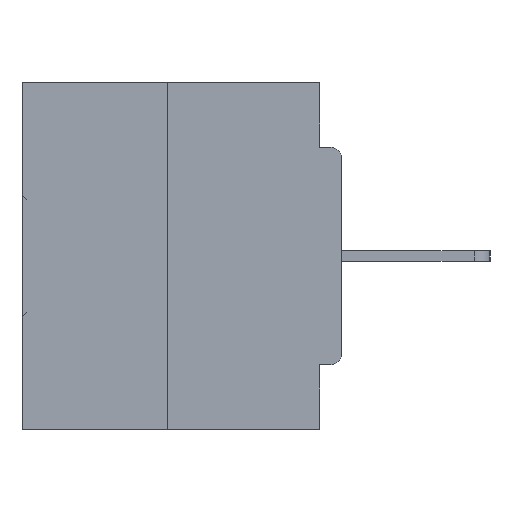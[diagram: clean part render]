
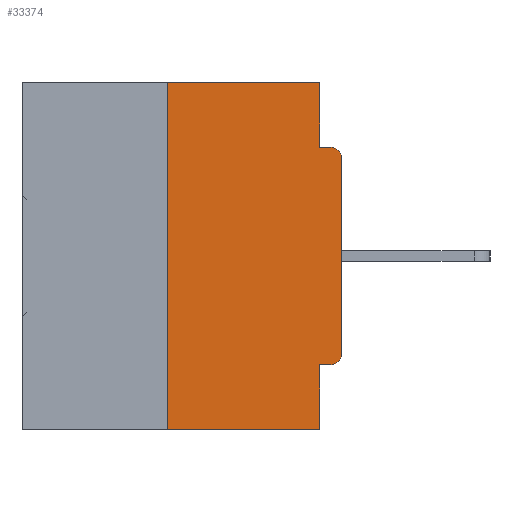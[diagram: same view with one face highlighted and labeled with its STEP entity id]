
A CAD part, left-side view. The second image highlights one B-rep face of the part: STEP entity #33374.
In plain terms, the highlighted planar face has unit normal (-1, 0, 0).
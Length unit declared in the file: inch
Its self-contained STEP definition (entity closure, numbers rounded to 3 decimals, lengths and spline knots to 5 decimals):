
#605 = LINE ( 'NONE', #21622, #7259 ) ;
#720 = EDGE_LOOP ( 'NONE', ( #32181, #9084, #12952, #34622, #1567, #32284, #33126, #6703, #37884, #9735 ) ) ;
#1174 = AXIS2_PLACEMENT_3D ( 'NONE', #32685, #8380, #14907 ) ;
#1273 = EDGE_CURVE ( 'NONE', #7712, #2412, #1544, .T. ) ;
#1544 = LINE ( 'NONE', #19913, #4070 ) ;
#1567 = ORIENTED_EDGE ( 'NONE', *, *, #1273, .F. ) ;
#2412 = VERTEX_POINT ( 'NONE', #40136 ) ;
#3053 = DIRECTION ( 'NONE',  ( 0., 0., -1. ) ) ;
#3484 = VERTEX_POINT ( 'NONE', #8749 ) ;
#3762 = CARTESIAN_POINT ( 'NONE',  ( 0., 0., 0. ) ) ;
#4070 = VECTOR ( 'NONE', #16831, 39.37008 ) ;
#6509 = CARTESIAN_POINT ( 'NONE',  ( 0., 0.031, 0. ) ) ;
#6703 = ORIENTED_EDGE ( 'NONE', *, *, #16996, .T. ) ;
#6751 = VERTEX_POINT ( 'NONE', #17397 ) ;
#7259 = VECTOR ( 'NONE', #18579, 39.37008 ) ;
#7712 = VERTEX_POINT ( 'NONE', #39703 ) ;
#8380 = DIRECTION ( 'NONE',  ( -1., 0., 0. ) ) ;
#8749 = CARTESIAN_POINT ( 'NONE',  ( 0., 0., -0.3915 ) ) ;
#9084 = ORIENTED_EDGE ( 'NONE', *, *, #36706, .F. ) ;
#9555 = CARTESIAN_POINT ( 'NONE',  ( 0., 0.031, -0.0935 ) ) ;
#9604 = VERTEX_POINT ( 'NONE', #22914 ) ;
#9735 = ORIENTED_EDGE ( 'NONE', *, *, #13893, .F. ) ;
#10556 = LINE ( 'NONE', #32204, #13340 ) ;
#11537 = EDGE_CURVE ( 'NONE', #32948, #9604, #605, .T. ) ;
#11586 = CIRCLE ( 'NONE', #1174, 0.015 ) ;
#12824 = CARTESIAN_POINT ( 'NONE',  ( 0., 0.25, -0.5 ) ) ;
#12952 = ORIENTED_EDGE ( 'NONE', *, *, #31692, .T. ) ;
#13172 = DIRECTION ( 'NONE',  ( 0., 0., -1. ) ) ;
#13340 = VECTOR ( 'NONE', #29141, 39.37008 ) ;
#13431 = CARTESIAN_POINT ( 'NONE',  ( 0., 0., -0.1085 ) ) ;
#13893 = EDGE_CURVE ( 'NONE', #32528, #32948, #37112, .T. ) ;
#14907 = DIRECTION ( 'NONE',  ( 0., 0., -1. ) ) ;
#16831 = DIRECTION ( 'NONE',  ( 0., 1., 0. ) ) ;
#16996 = EDGE_CURVE ( 'NONE', #30721, #9604, #26269, .T. ) ;
#17397 = CARTESIAN_POINT ( 'NONE',  ( 0., 0.25, 0. ) ) ;
#18256 = EDGE_CURVE ( 'NONE', #6751, #32528, #10556, .T. ) ;
#18538 = VECTOR ( 'NONE', #19283, 39.37008 ) ;
#18579 = DIRECTION ( 'NONE',  ( 0., -1., 0. ) ) ;
#18595 = VECTOR ( 'NONE', #35628, 39.37008 ) ;
#18772 = CARTESIAN_POINT ( 'NONE',  ( 0., 0.031, -0.5 ) ) ;
#19105 = FACE_OUTER_BOUND ( 'NONE', #720, .T. ) ;
#19249 = CARTESIAN_POINT ( 'NONE',  ( 0., 0.031, 0. ) ) ;
#19283 = DIRECTION ( 'NONE',  ( 0., 0., 1. ) ) ;
#19913 = CARTESIAN_POINT ( 'NONE',  ( 0., 0., -0.4065 ) ) ;
#20514 = EDGE_CURVE ( 'NONE', #3484, #30721, #31716, .T. ) ;
#21591 = DIRECTION ( 'NONE',  ( -1., 0., 0. ) ) ;
#21622 = CARTESIAN_POINT ( 'NONE',  ( 0., 0., -0.0935 ) ) ;
#21948 = DIRECTION ( 'NONE',  ( 0., 0., -1. ) ) ;
#22355 = DIRECTION ( 'NONE',  ( 1., 0., 0. ) ) ;
#22731 = VERTEX_POINT ( 'NONE', #12824 ) ;
#22914 = CARTESIAN_POINT ( 'NONE',  ( 0., 0.015, -0.0935 ) ) ;
#23186 = CARTESIAN_POINT ( 'NONE',  ( 0., 0.031, -0.5 ) ) ;
#24171 = VECTOR ( 'NONE', #3053, 39.37008 ) ;
#25467 = CARTESIAN_POINT ( 'NONE',  ( 0., 0.46, -0.5 ) ) ;
#25488 = VECTOR ( 'NONE', #37896, 39.37008 ) ;
#26269 = CIRCLE ( 'NONE', #29533, 0.015 ) ;
#26935 = DIRECTION ( 'NONE',  ( 0., 0., 1. ) ) ;
#29141 = DIRECTION ( 'NONE',  ( 0., -1., 0. ) ) ;
#29303 = LINE ( 'NONE', #23186, #18595 ) ;
#29533 = AXIS2_PLACEMENT_3D ( 'NONE', #36689, #21591, #13172 ) ;
#29544 = AXIS2_PLACEMENT_3D ( 'NONE', #38067, #22355, #21948 ) ;
#30182 = VERTEX_POINT ( 'NONE', #18772 ) ;
#30721 = VERTEX_POINT ( 'NONE', #13431 ) ;
#31692 = EDGE_CURVE ( 'NONE', #22731, #30182, #38114, .T. ) ;
#31716 = LINE ( 'NONE', #3762, #18538 ) ;
#32181 = ORIENTED_EDGE ( 'NONE', *, *, #18256, .F. ) ;
#32204 = CARTESIAN_POINT ( 'NONE',  ( 0., 0.46, 0. ) ) ;
#32284 = ORIENTED_EDGE ( 'NONE', *, *, #40044, .T. ) ;
#32528 = VERTEX_POINT ( 'NONE', #19249 ) ;
#32685 = CARTESIAN_POINT ( 'NONE',  ( 0., 0.015, -0.3915 ) ) ;
#32863 = CARTESIAN_POINT ( 'NONE',  ( 0., 0.25, 0. ) ) ;
#32948 = VERTEX_POINT ( 'NONE', #9555 ) ;
#33054 = LINE ( 'NONE', #32863, #36116 ) ;
#33126 = ORIENTED_EDGE ( 'NONE', *, *, #20514, .T. ) ;
#33374 = ADVANCED_FACE ( 'NONE', ( #19105 ), #34812, .F. ) ;
#34622 = ORIENTED_EDGE ( 'NONE', *, *, #38875, .F. ) ;
#34812 = PLANE ( 'NONE',  #29544 ) ;
#35628 = DIRECTION ( 'NONE',  ( 0., 0., -1. ) ) ;
#36116 = VECTOR ( 'NONE', #26935, 39.37008 ) ;
#36689 = CARTESIAN_POINT ( 'NONE',  ( 0., 0.015, -0.1085 ) ) ;
#36706 = EDGE_CURVE ( 'NONE', #22731, #6751, #33054, .T. ) ;
#37112 = LINE ( 'NONE', #6509, #24171 ) ;
#37884 = ORIENTED_EDGE ( 'NONE', *, *, #11537, .F. ) ;
#37896 = DIRECTION ( 'NONE',  ( 0., -1., 0. ) ) ;
#38067 = CARTESIAN_POINT ( 'NONE',  ( 0., 0.46, 0. ) ) ;
#38114 = LINE ( 'NONE', #25467, #25488 ) ;
#38875 = EDGE_CURVE ( 'NONE', #2412, #30182, #29303, .T. ) ;
#39703 = CARTESIAN_POINT ( 'NONE',  ( 0., 0.015, -0.4065 ) ) ;
#40044 = EDGE_CURVE ( 'NONE', #7712, #3484, #11586, .T. ) ;
#40136 = CARTESIAN_POINT ( 'NONE',  ( 0., 0.031, -0.4065 ) ) ;
